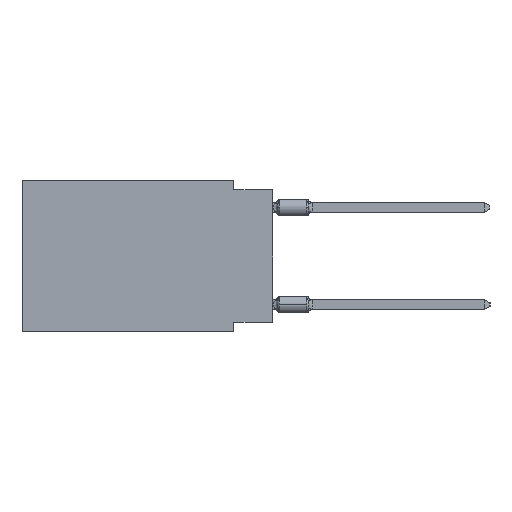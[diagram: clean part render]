
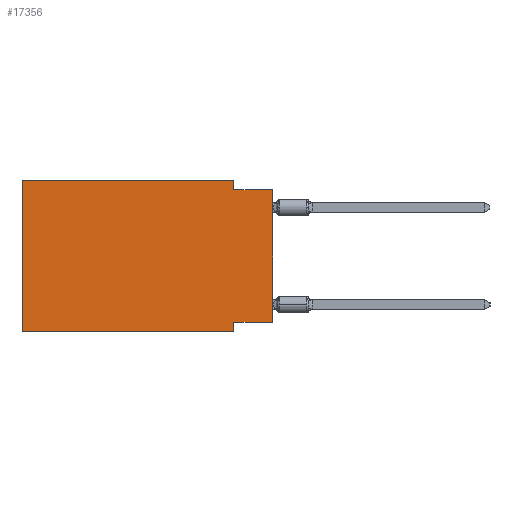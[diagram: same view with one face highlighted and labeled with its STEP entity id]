
A CAD part, left-side view. The second image highlights one B-rep face of the part: STEP entity #17356.
In plain terms, the highlighted planar face has unit normal (-1, 0, 0).
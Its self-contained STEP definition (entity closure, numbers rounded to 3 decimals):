
#1803 = EDGE_CURVE ( 'NONE', #26715, #14505, #1952, .T. ) ;
#1952 = LINE ( 'NONE', #7176, #8523 ) ;
#2208 = DIRECTION ( 'NONE',  ( 0., -1., 0. ) ) ;
#3295 = DIRECTION ( 'NONE',  ( 0., -1., 0. ) ) ;
#3468 = EDGE_CURVE ( 'NONE', #14505, #34103, #14392, .T. ) ;
#3722 = VECTOR ( 'NONE', #2208, 1000. ) ;
#3766 = ORIENTED_EDGE ( 'NONE', *, *, #11653, .T. ) ;
#4332 = ORIENTED_EDGE ( 'NONE', *, *, #3468, .F. ) ;
#4564 = ORIENTED_EDGE ( 'NONE', *, *, #18280, .F. ) ;
#4634 = PLANE ( 'NONE',  #10562 ) ;
#4894 = EDGE_CURVE ( 'NONE', #7540, #4959, #9256, .T. ) ;
#4898 = VECTOR ( 'NONE', #3295, 1000. ) ;
#4959 = VERTEX_POINT ( 'NONE', #7627 ) ;
#5863 = DIRECTION ( 'NONE',  ( 0., -1., 0. ) ) ;
#6038 = ORIENTED_EDGE ( 'NONE', *, *, #1803, .F. ) ;
#6857 = CARTESIAN_POINT ( 'NONE',  ( 0., 2.54, 0. ) ) ;
#7176 = CARTESIAN_POINT ( 'NONE',  ( 0., 2.54, 0. ) ) ;
#7540 = VERTEX_POINT ( 'NONE', #24874 ) ;
#7627 = CARTESIAN_POINT ( 'NONE',  ( 0., 2.54, -9.271 ) ) ;
#7776 = EDGE_CURVE ( 'NONE', #4959, #29778, #9803, .T. ) ;
#8523 = VECTOR ( 'NONE', #31343, 1000. ) ;
#9256 = LINE ( 'NONE', #25876, #26698 ) ;
#9803 = LINE ( 'NONE', #28607, #15554 ) ;
#10395 = ORIENTED_EDGE ( 'NONE', *, *, #4894, .F. ) ;
#10562 = AXIS2_PLACEMENT_3D ( 'NONE', #15540, #23085, #26463 ) ;
#10819 = LINE ( 'NONE', #13493, #3722 ) ;
#11213 = LINE ( 'NONE', #22137, #26846 ) ;
#11653 = EDGE_CURVE ( 'NONE', #17266, #29778, #11213, .T. ) ;
#12260 = DIRECTION ( 'NONE',  ( 0., 1., 0. ) ) ;
#12481 = CARTESIAN_POINT ( 'NONE',  ( 0., 0., 0. ) ) ;
#12502 = CARTESIAN_POINT ( 'NONE',  ( 0., 16.383, -9.906 ) ) ;
#13015 = LINE ( 'NONE', #12481, #13712 ) ;
#13493 = CARTESIAN_POINT ( 'NONE',  ( 0., 16.383, 0. ) ) ;
#13712 = VECTOR ( 'NONE', #16074, 1000. ) ;
#13859 = CARTESIAN_POINT ( 'NONE',  ( 0., 0., -0.635 ) ) ;
#14392 = LINE ( 'NONE', #13859, #4898 ) ;
#14505 = VERTEX_POINT ( 'NONE', #21472 ) ;
#14933 = CARTESIAN_POINT ( 'NONE',  ( 0., 0., -0.635 ) ) ;
#15494 = EDGE_LOOP ( 'NONE', ( #17923, #4332, #6038, #4564, #34576, #3766, #21548, #10395 ) ) ;
#15540 = CARTESIAN_POINT ( 'NONE',  ( 0., 16.383, 0. ) ) ;
#15554 = VECTOR ( 'NONE', #34846, 1000. ) ;
#16074 = DIRECTION ( 'NONE',  ( 0., 0., 1. ) ) ;
#17266 = VERTEX_POINT ( 'NONE', #12502 ) ;
#17356 = ADVANCED_FACE ( 'NONE', ( #29155 ), #4634, .F. ) ;
#17923 = ORIENTED_EDGE ( 'NONE', *, *, #31164, .T. ) ;
#18280 = EDGE_CURVE ( 'NONE', #25790, #26715, #10819, .T. ) ;
#20952 = CARTESIAN_POINT ( 'NONE',  ( 0., 2.54, -9.906 ) ) ;
#21472 = CARTESIAN_POINT ( 'NONE',  ( 0., 2.54, -0.635 ) ) ;
#21548 = ORIENTED_EDGE ( 'NONE', *, *, #7776, .F. ) ;
#21865 = CARTESIAN_POINT ( 'NONE',  ( 0., 16.383, 0. ) ) ;
#22137 = CARTESIAN_POINT ( 'NONE',  ( 0., 16.383, -9.906 ) ) ;
#23085 = DIRECTION ( 'NONE',  ( 1., 0., 0. ) ) ;
#24548 = LINE ( 'NONE', #21865, #30570 ) ;
#24874 = CARTESIAN_POINT ( 'NONE',  ( 0., 0., -9.271 ) ) ;
#24897 = EDGE_CURVE ( 'NONE', #17266, #25790, #24548, .T. ) ;
#25790 = VERTEX_POINT ( 'NONE', #32331 ) ;
#25876 = CARTESIAN_POINT ( 'NONE',  ( 0., 0., -9.271 ) ) ;
#26463 = DIRECTION ( 'NONE',  ( 0., 0., -1. ) ) ;
#26698 = VECTOR ( 'NONE', #12260, 1000. ) ;
#26715 = VERTEX_POINT ( 'NONE', #6857 ) ;
#26846 = VECTOR ( 'NONE', #5863, 1000. ) ;
#28607 = CARTESIAN_POINT ( 'NONE',  ( 0., 2.54, -9.906 ) ) ;
#29155 = FACE_OUTER_BOUND ( 'NONE', #15494, .T. ) ;
#29778 = VERTEX_POINT ( 'NONE', #20952 ) ;
#30570 = VECTOR ( 'NONE', #32776, 1000. ) ;
#31164 = EDGE_CURVE ( 'NONE', #7540, #34103, #13015, .T. ) ;
#31343 = DIRECTION ( 'NONE',  ( 0., 0., -1. ) ) ;
#32331 = CARTESIAN_POINT ( 'NONE',  ( 0., 16.383, 0. ) ) ;
#32776 = DIRECTION ( 'NONE',  ( 0., 0., 1. ) ) ;
#34103 = VERTEX_POINT ( 'NONE', #14933 ) ;
#34576 = ORIENTED_EDGE ( 'NONE', *, *, #24897, .F. ) ;
#34846 = DIRECTION ( 'NONE',  ( 0., 0., -1. ) ) ;
